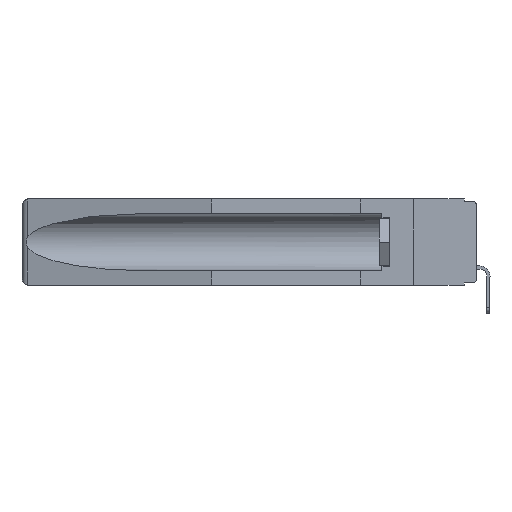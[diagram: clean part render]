
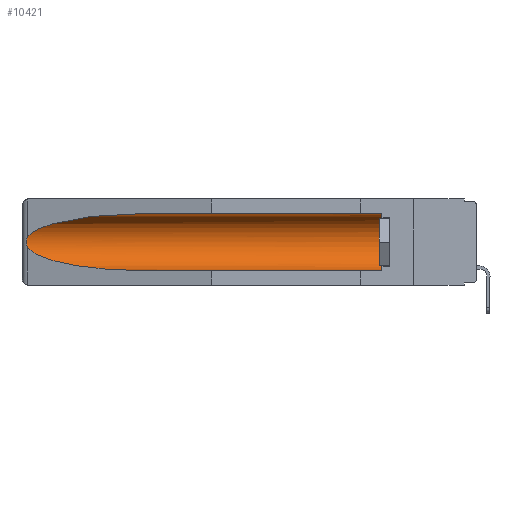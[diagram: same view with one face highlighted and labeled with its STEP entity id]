
A CAD part, left-side view. The second image highlights one B-rep face of the part: STEP entity #10421.
In plain terms, the highlighted cylindrical face has radius 2.857 mm (diameter 5.715 mm), a partial arc.
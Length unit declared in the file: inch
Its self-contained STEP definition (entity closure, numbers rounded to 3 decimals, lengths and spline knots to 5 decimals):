
#517 = DIRECTION ( 'NONE',  ( 0., 1., 0. ) ) ;
#1492 = CARTESIAN_POINT ( 'NONE',  ( 0.26537, 1.52718, -0.19328 ) ) ;
#1676 = VECTOR ( 'NONE', #3283, 39.37008 ) ;
#1707 =( BOUNDED_CURVE ( )  B_SPLINE_CURVE ( 3, ( #4520, #19695, #11248, #6198 ),
 .UNSPECIFIED., .F., .T. ) 
 B_SPLINE_CURVE_WITH_KNOTS ( ( 4, 4 ),
 ( 0.1948, 1.5708 ),
 .UNSPECIFIED. ) 
 CURVE ( )  GEOMETRIC_REPRESENTATION_ITEM ( )  RATIONAL_B_SPLINE_CURVE ( ( 1., 0.848, 0.848, 1. ) ) 
 REPRESENTATION_ITEM ( '' )  );
#1863 = FACE_OUTER_BOUND ( 'NONE', #10343, .T. ) ;
#1929 = AXIS2_PLACEMENT_3D ( 'NONE', #9147, #517, #19163 ) ;
#2849 = VERTEX_POINT ( 'NONE', #11005 ) ;
#3050 = CARTESIAN_POINT ( 'NONE',  ( 0.26597, 1.52961, -0.15275 ) ) ;
#3283 = DIRECTION ( 'NONE',  ( 0., 1., 0. ) ) ;
#4398 =( BOUNDED_CURVE ( )  B_SPLINE_CURVE ( 3, ( #14555, #6272, #16159, #16230 ),
 .UNSPECIFIED., .F., .F. ) 
 B_SPLINE_CURVE_WITH_KNOTS ( ( 4, 4 ),
 ( 4.71239, 6.08839 ),
 .UNSPECIFIED. ) 
 CURVE ( )  GEOMETRIC_REPRESENTATION_ITEM ( )  RATIONAL_B_SPLINE_CURVE ( ( 1., 0.848, 0.848, 1. ) ) 
 REPRESENTATION_ITEM ( '' )  );
#4520 = CARTESIAN_POINT ( 'NONE',  ( 0.26537, 1.52718, -0.19328 ) ) ;
#4577 = CARTESIAN_POINT ( 'NONE',  ( 0.155, -0.30754, -0.284 ) ) ;
#4735 = CARTESIAN_POINT ( 'NONE',  ( 0.2675, 1.53308, -0.16763 ) ) ;
#4827 = EDGE_CURVE ( 'NONE', #20857, #9343, #19462, .T. ) ;
#5038 = ORIENTED_EDGE ( 'NONE', *, *, #13027, .T. ) ;
#6107 = EDGE_CURVE ( 'NONE', #15120, #15303, #21526, .T. ) ;
#6198 = CARTESIAN_POINT ( 'NONE',  ( 0.155, 1.07973, -0.284 ) ) ;
#6272 = CARTESIAN_POINT ( 'NONE',  ( 0.21114, 1.30732, -0.059 ) ) ;
#6420 = CARTESIAN_POINT ( 'NONE',  ( 0.2675, 1.53308, -0.17534 ) ) ;
#6953 = EDGE_CURVE ( 'NONE', #2849, #16717, #7612, .T. ) ;
#7400 = ORIENTED_EDGE ( 'NONE', *, *, #7949, .T. ) ;
#7411 = CARTESIAN_POINT ( 'NONE',  ( 0.26537, 1.52718, -0.19328 ) ) ;
#7612 = B_SPLINE_CURVE_WITH_KNOTS ( 'NONE', 3,
 ( #19705, #3050, #12945, #13086, #4735, #6420, #19778, #9779, #21489, #1492 ),
 .UNSPECIFIED., .F., .F.,
 ( 4, 2, 2, 2, 4 ),
 ( 0., 0.00029, 0.00058, 0.00087, 0.00117 ),
 .UNSPECIFIED. ) ;
#7621 = CYLINDRICAL_SURFACE ( 'NONE', #1929, 0.1125 ) ;
#7733 = CARTESIAN_POINT ( 'NONE',  ( 0.155, 0.126, -0.1715 ) ) ;
#7933 = DIRECTION ( 'NONE',  ( 0., 1., 0. ) ) ;
#7949 = EDGE_CURVE ( 'NONE', #9343, #2849, #4398, .T. ) ;
#9147 = CARTESIAN_POINT ( 'NONE',  ( 0.155, -0.30754, -0.1715 ) ) ;
#9343 = VERTEX_POINT ( 'NONE', #14574 ) ;
#9779 = CARTESIAN_POINT ( 'NONE',  ( 0.26655, 1.53094, -0.18657 ) ) ;
#10343 = EDGE_LOOP ( 'NONE', ( #7400, #14794, #13690, #14246, #5038, #15025 ) ) ;
#10421 = ADVANCED_FACE ( 'NONE', ( #1863 ), #7621, .F. ) ;
#11005 = CARTESIAN_POINT ( 'NONE',  ( 0.26537, 1.52718, -0.14972 ) ) ;
#11109 = DIRECTION ( 'NONE',  ( 0., 0., 1. ) ) ;
#11248 = CARTESIAN_POINT ( 'NONE',  ( 0.21114, 1.30732, -0.284 ) ) ;
#12219 = AXIS2_PLACEMENT_3D ( 'NONE', #7733, #16070, #11109 ) ;
#12945 = CARTESIAN_POINT ( 'NONE',  ( 0.26654, 1.53092, -0.15636 ) ) ;
#13027 = EDGE_CURVE ( 'NONE', #15120, #20857, #19019, .T. ) ;
#13086 = CARTESIAN_POINT ( 'NONE',  ( 0.2673, 1.5327, -0.16383 ) ) ;
#13687 = VECTOR ( 'NONE', #7933, 39.37008 ) ;
#13690 = ORIENTED_EDGE ( 'NONE', *, *, #16384, .T. ) ;
#14246 = ORIENTED_EDGE ( 'NONE', *, *, #6107, .F. ) ;
#14555 = CARTESIAN_POINT ( 'NONE',  ( 0.155, 1.07973, -0.059 ) ) ;
#14574 = CARTESIAN_POINT ( 'NONE',  ( 0.155, 1.07973, -0.059 ) ) ;
#14794 = ORIENTED_EDGE ( 'NONE', *, *, #6953, .T. ) ;
#15025 = ORIENTED_EDGE ( 'NONE', *, *, #4827, .T. ) ;
#15120 = VERTEX_POINT ( 'NONE', #20435 ) ;
#15199 = CARTESIAN_POINT ( 'NONE',  ( 0.155, -0.30754, -0.059 ) ) ;
#15303 = VERTEX_POINT ( 'NONE', #20139 ) ;
#16070 = DIRECTION ( 'NONE',  ( 0., -1., 0. ) ) ;
#16159 = CARTESIAN_POINT ( 'NONE',  ( 0.25451, 1.48313, -0.09465 ) ) ;
#16230 = CARTESIAN_POINT ( 'NONE',  ( 0.26537, 1.52718, -0.14972 ) ) ;
#16384 = EDGE_CURVE ( 'NONE', #16717, #15303, #1707, .T. ) ;
#16717 = VERTEX_POINT ( 'NONE', #7411 ) ;
#18031 = CARTESIAN_POINT ( 'NONE',  ( 0.155, 0.126, -0.059 ) ) ;
#19019 = CIRCLE ( 'NONE', #12219, 0.1125 ) ;
#19163 = DIRECTION ( 'NONE',  ( 0., 0., 1. ) ) ;
#19462 = LINE ( 'NONE', #15199, #1676 ) ;
#19695 = CARTESIAN_POINT ( 'NONE',  ( 0.25451, 1.48313, -0.24835 ) ) ;
#19705 = CARTESIAN_POINT ( 'NONE',  ( 0.26537, 1.52718, -0.14972 ) ) ;
#19778 = CARTESIAN_POINT ( 'NONE',  ( 0.2673, 1.53269, -0.17917 ) ) ;
#20139 = CARTESIAN_POINT ( 'NONE',  ( 0.155, 1.07973, -0.284 ) ) ;
#20435 = CARTESIAN_POINT ( 'NONE',  ( 0.155, 0.126, -0.284 ) ) ;
#20857 = VERTEX_POINT ( 'NONE', #18031 ) ;
#21489 = CARTESIAN_POINT ( 'NONE',  ( 0.26597, 1.5296, -0.19026 ) ) ;
#21526 = LINE ( 'NONE', #4577, #13687 ) ;
